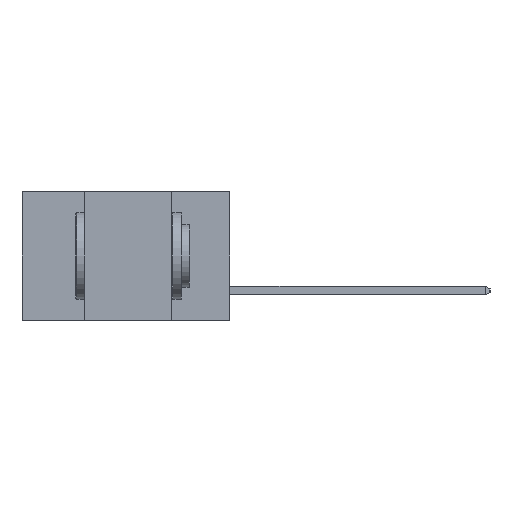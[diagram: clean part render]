
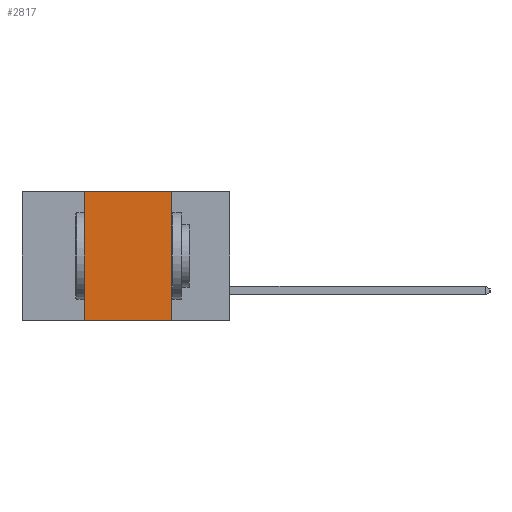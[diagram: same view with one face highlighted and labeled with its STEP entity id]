
A CAD part, left-side view. The second image highlights one B-rep face of the part: STEP entity #2817.
In plain terms, the highlighted planar face has unit normal (-1, 0, 0).
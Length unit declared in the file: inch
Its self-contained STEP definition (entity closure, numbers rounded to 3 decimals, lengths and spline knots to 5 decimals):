
#224 = CARTESIAN_POINT ( 'NONE',  ( 0., 0.17, -0.37 ) ) ;
#440 = VERTEX_POINT ( 'NONE', #15691 ) ;
#835 = FACE_OUTER_BOUND ( 'NONE', #16484, .T. ) ;
#1221 = CARTESIAN_POINT ( 'NONE',  ( 0., 0.17, 0. ) ) ;
#2097 = LINE ( 'NONE', #10430, #15733 ) ;
#2132 = DIRECTION ( 'NONE',  ( 0., 0., -1. ) ) ;
#2158 = DIRECTION ( 'NONE',  ( 1., 0., 0. ) ) ;
#2370 = CARTESIAN_POINT ( 'NONE',  ( 0., 0.6, 0. ) ) ;
#2426 = PLANE ( 'NONE',  #10997 ) ;
#2817 = ADVANCED_FACE ( 'NONE', ( #835 ), #2426, .F. ) ;
#3776 = VECTOR ( 'NONE', #7566, 39.37008 ) ;
#3944 = VERTEX_POINT ( 'NONE', #3970 ) ;
#3970 = CARTESIAN_POINT ( 'NONE',  ( 0., 0.42, 0. ) ) ;
#3989 = DIRECTION ( 'NONE',  ( 0., 0., -1. ) ) ;
#4996 = VERTEX_POINT ( 'NONE', #1221 ) ;
#6222 = VERTEX_POINT ( 'NONE', #224 ) ;
#6282 = ORIENTED_EDGE ( 'NONE', *, *, #9750, .F. ) ;
#6399 = DIRECTION ( 'NONE',  ( 0., 0., 1. ) ) ;
#7566 = DIRECTION ( 'NONE',  ( 0., -1., 0. ) ) ;
#7682 = LINE ( 'NONE', #11459, #10690 ) ;
#8734 = DIRECTION ( 'NONE',  ( 0., -1., 0. ) ) ;
#8813 = EDGE_CURVE ( 'NONE', #440, #3944, #7682, .T. ) ;
#8910 = EDGE_CURVE ( 'NONE', #4996, #6222, #2097, .T. ) ;
#9319 = ORIENTED_EDGE ( 'NONE', *, *, #8813, .F. ) ;
#9750 = EDGE_CURVE ( 'NONE', #3944, #4996, #15702, .T. ) ;
#10430 = CARTESIAN_POINT ( 'NONE',  ( 0., 0.17, -0.37 ) ) ;
#10690 = VECTOR ( 'NONE', #6399, 39.37008 ) ;
#10997 = AXIS2_PLACEMENT_3D ( 'NONE', #2370, #2158, #2132 ) ;
#11459 = CARTESIAN_POINT ( 'NONE',  ( 0., 0.42, -0.37 ) ) ;
#12010 = VECTOR ( 'NONE', #8734, 39.37008 ) ;
#12258 = ORIENTED_EDGE ( 'NONE', *, *, #16300, .T. ) ;
#13028 = ORIENTED_EDGE ( 'NONE', *, *, #8910, .F. ) ;
#13572 = LINE ( 'NONE', #15077, #3776 ) ;
#14945 = CARTESIAN_POINT ( 'NONE',  ( 0., 0.6, 0. ) ) ;
#15077 = CARTESIAN_POINT ( 'NONE',  ( 0., 0.6, -0.37 ) ) ;
#15691 = CARTESIAN_POINT ( 'NONE',  ( 0., 0.42, -0.37 ) ) ;
#15702 = LINE ( 'NONE', #14945, #12010 ) ;
#15733 = VECTOR ( 'NONE', #3989, 39.37008 ) ;
#16300 = EDGE_CURVE ( 'NONE', #440, #6222, #13572, .T. ) ;
#16484 = EDGE_LOOP ( 'NONE', ( #13028, #6282, #9319, #12258 ) ) ;
